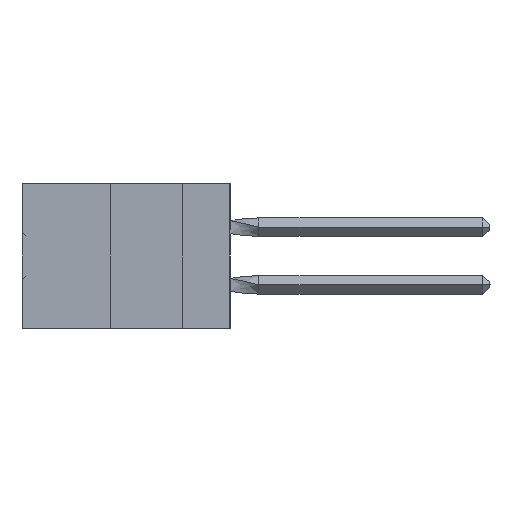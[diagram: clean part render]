
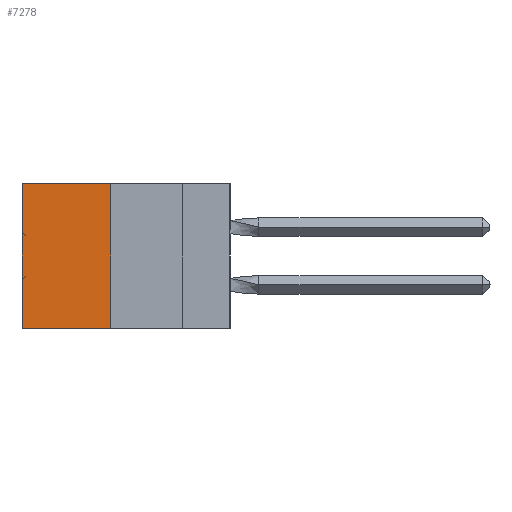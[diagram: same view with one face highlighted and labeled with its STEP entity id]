
A CAD part, left-side view. The second image highlights one B-rep face of the part: STEP entity #7278.
In plain terms, the highlighted planar face has unit normal (-1, 0, 0).
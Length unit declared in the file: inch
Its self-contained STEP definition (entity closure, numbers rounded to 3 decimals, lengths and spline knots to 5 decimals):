
#3674 = DIRECTION ( 'NONE',  ( 0., 1., 0. ) ) ;
#7278 = ADVANCED_FACE ( 'NONE', ( #10280 ), #36546, .F. ) ;
#10280 = FACE_OUTER_BOUND ( 'NONE', #22687, .T. ) ;
#12852 = VECTOR ( 'NONE', #55377, 39.37008 ) ;
#14831 = EDGE_CURVE ( 'NONE', #48783, #48607, #36931, .T. ) ;
#15370 = DIRECTION ( 'NONE',  ( 0., 1., 0. ) ) ;
#17571 = ORIENTED_EDGE ( 'NONE', *, *, #47904, .T. ) ;
#18980 = EDGE_CURVE ( 'NONE', #34734, #48607, #22405, .T. ) ;
#22405 = LINE ( 'NONE', #57346, #42603 ) ;
#22687 = EDGE_LOOP ( 'NONE', ( #39574, #36021, #32261, #17571 ) ) ;
#22719 = CARTESIAN_POINT ( 'NONE',  ( 0.305, 0.413, -0.5 ) ) ;
#23941 = VERTEX_POINT ( 'NONE', #52582 ) ;
#31287 = CARTESIAN_POINT ( 'NONE',  ( 0.305, 0.413, -0.5 ) ) ;
#32127 = DIRECTION ( 'NONE',  ( 1., 0., 0. ) ) ;
#32261 = ORIENTED_EDGE ( 'NONE', *, *, #32995, .F. ) ;
#32995 = EDGE_CURVE ( 'NONE', #23941, #48783, #43493, .T. ) ;
#34734 = VERTEX_POINT ( 'NONE', #46006 ) ;
#36021 = ORIENTED_EDGE ( 'NONE', *, *, #14831, .F. ) ;
#36546 = PLANE ( 'NONE',  #57932 ) ;
#36931 = LINE ( 'NONE', #44358, #48139 ) ;
#39574 = ORIENTED_EDGE ( 'NONE', *, *, #18980, .T. ) ;
#40754 = CARTESIAN_POINT ( 'NONE',  ( 0.305, 0.72, -0.5 ) ) ;
#41705 = LINE ( 'NONE', #60548, #43202 ) ;
#42603 = VECTOR ( 'NONE', #58171, 39.37008 ) ;
#43202 = VECTOR ( 'NONE', #3674, 39.37008 ) ;
#43493 = LINE ( 'NONE', #31287, #12852 ) ;
#44358 = CARTESIAN_POINT ( 'NONE',  ( 0.305, 0.413, -0.5 ) ) ;
#46006 = CARTESIAN_POINT ( 'NONE',  ( 0.305, 0.72, 0. ) ) ;
#47616 = CARTESIAN_POINT ( 'NONE',  ( 0.305, 0.413, -0.5 ) ) ;
#47904 = EDGE_CURVE ( 'NONE', #23941, #34734, #41705, .T. ) ;
#48139 = VECTOR ( 'NONE', #15370, 39.37008 ) ;
#48607 = VERTEX_POINT ( 'NONE', #40754 ) ;
#48783 = VERTEX_POINT ( 'NONE', #47616 ) ;
#52582 = CARTESIAN_POINT ( 'NONE',  ( 0.305, 0.413, 0. ) ) ;
#55377 = DIRECTION ( 'NONE',  ( 0., 0., -1. ) ) ;
#57346 = CARTESIAN_POINT ( 'NONE',  ( 0.305, 0.72, -0.5 ) ) ;
#57932 = AXIS2_PLACEMENT_3D ( 'NONE', #22719, #32127, #60405 ) ;
#58171 = DIRECTION ( 'NONE',  ( 0., 0., -1. ) ) ;
#60405 = DIRECTION ( 'NONE',  ( 0., 0., -1. ) ) ;
#60548 = CARTESIAN_POINT ( 'NONE',  ( 0.305, 0.413, 0. ) ) ;
